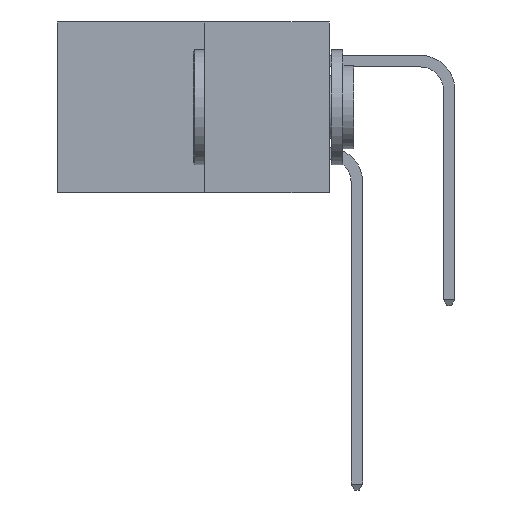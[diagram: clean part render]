
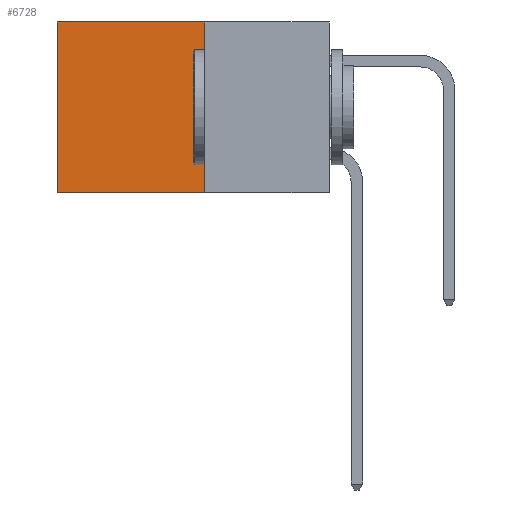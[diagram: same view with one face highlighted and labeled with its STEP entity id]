
A CAD part, left-side view. The second image highlights one B-rep face of the part: STEP entity #6728.
In plain terms, the highlighted planar face has unit normal (-1, 0, 0).
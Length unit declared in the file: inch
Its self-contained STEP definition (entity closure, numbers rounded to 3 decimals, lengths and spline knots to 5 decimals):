
#277 = VECTOR ( 'NONE', #5954, 39.37008 ) ;
#390 = EDGE_LOOP ( 'NONE', ( #7265, #4524, #7642, #9680 ) ) ;
#1212 = CARTESIAN_POINT ( 'NONE',  ( 0.277, 0.27, 0. ) ) ;
#1824 = VECTOR ( 'NONE', #4963, 39.37008 ) ;
#1853 = DIRECTION ( 'NONE',  ( 1., 0., 0. ) ) ;
#2487 = VECTOR ( 'NONE', #6137, 39.37008 ) ;
#2740 = LINE ( 'NONE', #5325, #2487 ) ;
#2888 = LINE ( 'NONE', #3294, #9008 ) ;
#3294 = CARTESIAN_POINT ( 'NONE',  ( 0.277, 0.27, -0.37 ) ) ;
#3793 = CARTESIAN_POINT ( 'NONE',  ( 0.277, 0.59, -0.37 ) ) ;
#3990 = VERTEX_POINT ( 'NONE', #9623 ) ;
#3998 = AXIS2_PLACEMENT_3D ( 'NONE', #5789, #1853, #7389 ) ;
#4257 = LINE ( 'NONE', #1212, #277 ) ;
#4524 = ORIENTED_EDGE ( 'NONE', *, *, #8850, .F. ) ;
#4601 = FACE_OUTER_BOUND ( 'NONE', #390, .T. ) ;
#4742 = EDGE_CURVE ( 'NONE', #6171, #5660, #6287, .T. ) ;
#4963 = DIRECTION ( 'NONE',  ( 0., 0., -1. ) ) ;
#5323 = CARTESIAN_POINT ( 'NONE',  ( 0.277, 0.27, 0. ) ) ;
#5325 = CARTESIAN_POINT ( 'NONE',  ( 0.277, 0.27, -0.37 ) ) ;
#5660 = VERTEX_POINT ( 'NONE', #3793 ) ;
#5789 = CARTESIAN_POINT ( 'NONE',  ( 0.277, 0.27, -0.37 ) ) ;
#5954 = DIRECTION ( 'NONE',  ( 0., 1., 0. ) ) ;
#6068 = EDGE_CURVE ( 'NONE', #7013, #6171, #4257, .T. ) ;
#6137 = DIRECTION ( 'NONE',  ( 0., 1., 0. ) ) ;
#6171 = VERTEX_POINT ( 'NONE', #10093 ) ;
#6287 = LINE ( 'NONE', #7341, #1824 ) ;
#6492 = EDGE_CURVE ( 'NONE', #7013, #3990, #2888, .T. ) ;
#6728 = ADVANCED_FACE ( 'NONE', ( #4601 ), #8999, .F. ) ;
#7013 = VERTEX_POINT ( 'NONE', #5323 ) ;
#7265 = ORIENTED_EDGE ( 'NONE', *, *, #4742, .T. ) ;
#7341 = CARTESIAN_POINT ( 'NONE',  ( 0.277, 0.59, -0.37 ) ) ;
#7389 = DIRECTION ( 'NONE',  ( 0., 0., -1. ) ) ;
#7642 = ORIENTED_EDGE ( 'NONE', *, *, #6492, .F. ) ;
#8056 = DIRECTION ( 'NONE',  ( 0., 0., -1. ) ) ;
#8850 = EDGE_CURVE ( 'NONE', #3990, #5660, #2740, .T. ) ;
#8999 = PLANE ( 'NONE',  #3998 ) ;
#9008 = VECTOR ( 'NONE', #8056, 39.37008 ) ;
#9623 = CARTESIAN_POINT ( 'NONE',  ( 0.277, 0.27, -0.37 ) ) ;
#9680 = ORIENTED_EDGE ( 'NONE', *, *, #6068, .T. ) ;
#10093 = CARTESIAN_POINT ( 'NONE',  ( 0.277, 0.59, 0. ) ) ;
